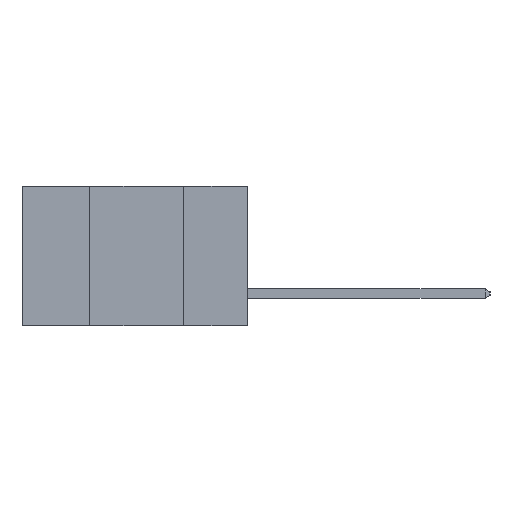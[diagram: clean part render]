
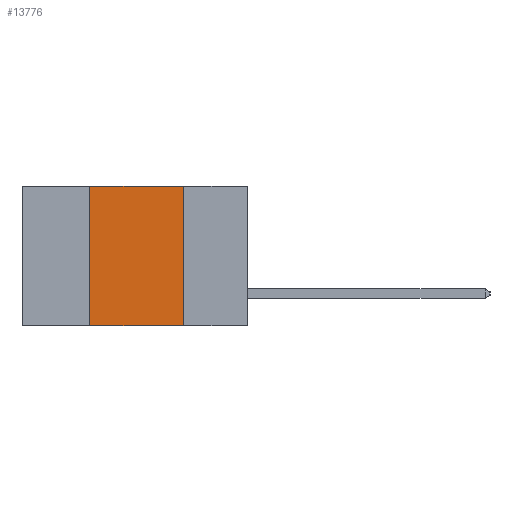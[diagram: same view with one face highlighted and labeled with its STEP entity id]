
A CAD part, left-side view. The second image highlights one B-rep face of the part: STEP entity #13776.
In plain terms, the highlighted planar face has unit normal (-1, 0, 0).
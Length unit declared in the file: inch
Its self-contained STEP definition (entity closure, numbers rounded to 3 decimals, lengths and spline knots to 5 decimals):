
#1438 = FACE_OUTER_BOUND ( 'NONE', #6273, .T. ) ;
#1591 = EDGE_CURVE ( 'NONE', #22487, #5255, #20286, .T. ) ;
#2257 = EDGE_CURVE ( 'NONE', #26670, #5255, #27100, .T. ) ;
#3939 = VERTEX_POINT ( 'NONE', #28366 ) ;
#4065 = DIRECTION ( 'NONE',  ( 0., -1., 0. ) ) ;
#5255 = VERTEX_POINT ( 'NONE', #28632 ) ;
#6273 = EDGE_LOOP ( 'NONE', ( #28983, #26301, #27864, #10516 ) ) ;
#7404 = VECTOR ( 'NONE', #4065, 39.37008 ) ;
#9004 = CARTESIAN_POINT ( 'NONE',  ( 0., 0.6, 0. ) ) ;
#9639 = CARTESIAN_POINT ( 'NONE',  ( 0., 0.6, -0.37 ) ) ;
#10516 = ORIENTED_EDGE ( 'NONE', *, *, #2257, .T. ) ;
#10767 = DIRECTION ( 'NONE',  ( 0., -1., 0. ) ) ;
#11260 = VECTOR ( 'NONE', #26032, 39.37008 ) ;
#11524 = DIRECTION ( 'NONE',  ( 0., 0., -1. ) ) ;
#12000 = VECTOR ( 'NONE', #10767, 39.37008 ) ;
#12144 = DIRECTION ( 'NONE',  ( 0., 0., -1. ) ) ;
#13520 = CARTESIAN_POINT ( 'NONE',  ( 0., 0.17, 0. ) ) ;
#13664 = VECTOR ( 'NONE', #12144, 39.37008 ) ;
#13748 = CARTESIAN_POINT ( 'NONE',  ( 0., 0.42, -0.37 ) ) ;
#13776 = ADVANCED_FACE ( 'NONE', ( #1438 ), #18718, .F. ) ;
#18718 = PLANE ( 'NONE',  #27417 ) ;
#20163 = EDGE_CURVE ( 'NONE', #26670, #3939, #30879, .T. ) ;
#20286 = LINE ( 'NONE', #31205, #13664 ) ;
#22487 = VERTEX_POINT ( 'NONE', #13520 ) ;
#25895 = EDGE_CURVE ( 'NONE', #3939, #22487, #31623, .T. ) ;
#26032 = DIRECTION ( 'NONE',  ( 0., 0., 1. ) ) ;
#26280 = DIRECTION ( 'NONE',  ( 1., 0., 0. ) ) ;
#26301 = ORIENTED_EDGE ( 'NONE', *, *, #25895, .F. ) ;
#26670 = VERTEX_POINT ( 'NONE', #13748 ) ;
#27100 = LINE ( 'NONE', #9639, #7404 ) ;
#27417 = AXIS2_PLACEMENT_3D ( 'NONE', #9004, #26280, #11524 ) ;
#27864 = ORIENTED_EDGE ( 'NONE', *, *, #20163, .F. ) ;
#27997 = CARTESIAN_POINT ( 'NONE',  ( 0., 0.6, 0. ) ) ;
#28366 = CARTESIAN_POINT ( 'NONE',  ( 0., 0.42, 0. ) ) ;
#28504 = CARTESIAN_POINT ( 'NONE',  ( 0., 0.42, 0. ) ) ;
#28632 = CARTESIAN_POINT ( 'NONE',  ( 0., 0.17, -0.37 ) ) ;
#28983 = ORIENTED_EDGE ( 'NONE', *, *, #1591, .F. ) ;
#30879 = LINE ( 'NONE', #28504, #11260 ) ;
#31205 = CARTESIAN_POINT ( 'NONE',  ( 0., 0.17, 0. ) ) ;
#31623 = LINE ( 'NONE', #27997, #12000 ) ;
